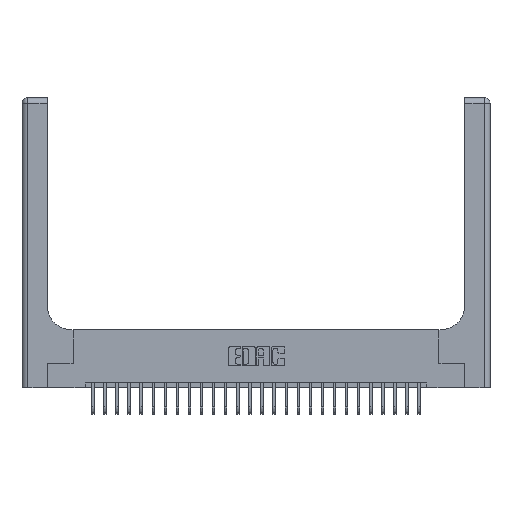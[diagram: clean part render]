
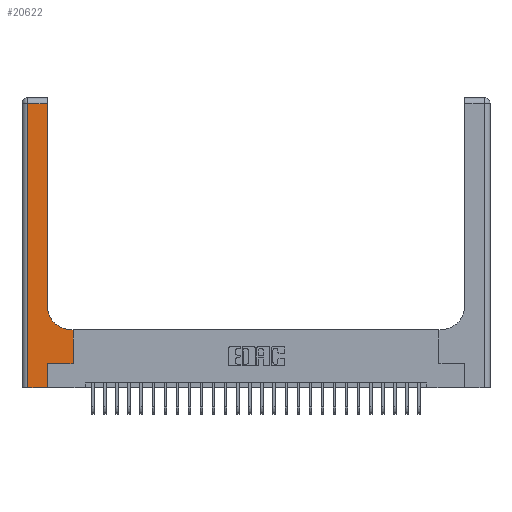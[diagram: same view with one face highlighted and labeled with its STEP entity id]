
A CAD part, top view. The second image highlights one B-rep face of the part: STEP entity #20622.
In plain terms, the highlighted planar face has unit normal (0, 0, 1).
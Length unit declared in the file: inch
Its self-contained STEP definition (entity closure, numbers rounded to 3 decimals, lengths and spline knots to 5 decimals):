
#846 = DIRECTION ( 'NONE',  ( 0., 1., 0. ) ) ;
#1114 = ORIENTED_EDGE ( 'NONE', *, *, #23028, .T. ) ;
#1119 = CARTESIAN_POINT ( 'NONE',  ( 0.528, 0.25, 0.37 ) ) ;
#1219 = VERTEX_POINT ( 'NONE', #4913 ) ;
#1459 = DIRECTION ( 'NONE',  ( -1., 0., 0. ) ) ;
#1529 = VECTOR ( 'NONE', #24369, 39.37008 ) ;
#1841 = CARTESIAN_POINT ( 'NONE',  ( 0.06, 3., 0.37 ) ) ;
#2082 = CARTESIAN_POINT ( 'NONE',  ( 0.528, 0.25, 0.37 ) ) ;
#2183 = AXIS2_PLACEMENT_3D ( 'NONE', #10645, #23799, #12576 ) ;
#2284 = LINE ( 'NONE', #24135, #16318 ) ;
#2545 = VERTEX_POINT ( 'NONE', #14846 ) ;
#2704 = AXIS2_PLACEMENT_3D ( 'NONE', #14211, #2793, #16126 ) ;
#2793 = DIRECTION ( 'NONE',  ( 0., 0., -1. ) ) ;
#3782 = DIRECTION ( 'NONE',  ( 0., -1., 0. ) ) ;
#3996 = EDGE_CURVE ( 'NONE', #2545, #10457, #22700, .T. ) ;
#4897 = CARTESIAN_POINT ( 'NONE',  ( 0.26, 0.85, 0.37 ) ) ;
#4913 = CARTESIAN_POINT ( 'NONE',  ( 0.06, 2.94, 0.37 ) ) ;
#5223 = ORIENTED_EDGE ( 'NONE', *, *, #15168, .T. ) ;
#5311 = LINE ( 'NONE', #9800, #19837 ) ;
#6964 = VECTOR ( 'NONE', #3782, 39.37008 ) ;
#7145 = FACE_OUTER_BOUND ( 'NONE', #19048, .T. ) ;
#7819 = CARTESIAN_POINT ( 'NONE',  ( 0.265, 0., 0.37 ) ) ;
#8802 = DIRECTION ( 'NONE',  ( 0., 1., 0. ) ) ;
#8806 = ORIENTED_EDGE ( 'NONE', *, *, #12854, .T. ) ;
#9182 = VECTOR ( 'NONE', #846, 39.37008 ) ;
#9800 = CARTESIAN_POINT ( 'NONE',  ( 0., 0., 0.37 ) ) ;
#10286 = VERTEX_POINT ( 'NONE', #23382 ) ;
#10457 = VERTEX_POINT ( 'NONE', #10545 ) ;
#10545 = CARTESIAN_POINT ( 'NONE',  ( 0.265, 0.25, 0.37 ) ) ;
#10645 = CARTESIAN_POINT ( 'NONE',  ( 0., 3., 0.37 ) ) ;
#11180 = CARTESIAN_POINT ( 'NONE',  ( 0.528, 0.6, 0.37 ) ) ;
#11387 = VERTEX_POINT ( 'NONE', #2082 ) ;
#11705 = VERTEX_POINT ( 'NONE', #18222 ) ;
#11707 = LINE ( 'NONE', #22487, #1529 ) ;
#12102 = LINE ( 'NONE', #16204, #16572 ) ;
#12576 = DIRECTION ( 'NONE',  ( -1., 0., 0. ) ) ;
#12854 = EDGE_CURVE ( 'NONE', #1219, #21657, #22038, .T. ) ;
#14211 = CARTESIAN_POINT ( 'NONE',  ( 0.51, 0.85, 0.37 ) ) ;
#14584 = EDGE_CURVE ( 'NONE', #11387, #23557, #16471, .T. ) ;
#14768 = EDGE_CURVE ( 'NONE', #10457, #11387, #11707, .T. ) ;
#14846 = CARTESIAN_POINT ( 'NONE',  ( 0.265, 0., 0.37 ) ) ;
#15168 = EDGE_CURVE ( 'NONE', #23996, #11705, #24209, .T. ) ;
#15738 = ORIENTED_EDGE ( 'NONE', *, *, #24145, .T. ) ;
#15866 = VECTOR ( 'NONE', #8802, 39.37008 ) ;
#16104 = CARTESIAN_POINT ( 'NONE',  ( 0.06, 0., 0.37 ) ) ;
#16126 = DIRECTION ( 'NONE',  ( 1., 0., 0. ) ) ;
#16204 = CARTESIAN_POINT ( 'NONE',  ( 0., 2.94, 0.37 ) ) ;
#16318 = VECTOR ( 'NONE', #1459, 39.37008 ) ;
#16471 = LINE ( 'NONE', #1119, #15866 ) ;
#16572 = VECTOR ( 'NONE', #18092, 39.37008 ) ;
#17132 = EDGE_CURVE ( 'NONE', #11705, #1219, #12102, .T. ) ;
#17168 = VECTOR ( 'NONE', #22909, 39.37008 ) ;
#17465 = DIRECTION ( 'NONE',  ( 1., 0., 0. ) ) ;
#18092 = DIRECTION ( 'NONE',  ( -1., 0., 0. ) ) ;
#18222 = CARTESIAN_POINT ( 'NONE',  ( 0.26, 2.94, 0.37 ) ) ;
#18322 = ORIENTED_EDGE ( 'NONE', *, *, #17132, .T. ) ;
#18592 = ORIENTED_EDGE ( 'NONE', *, *, #14584, .T. ) ;
#19048 = EDGE_LOOP ( 'NONE', ( #5223, #18322, #8806, #20365, #20625, #22366, #18592, #15738, #1114 ) ) ;
#19837 = VECTOR ( 'NONE', #17465, 39.37008 ) ;
#20116 = CIRCLE ( 'NONE', #2704, 0.25 ) ;
#20365 = ORIENTED_EDGE ( 'NONE', *, *, #22852, .T. ) ;
#20622 = ADVANCED_FACE ( 'NONE', ( #7145 ), #21936, .F. ) ;
#20625 = ORIENTED_EDGE ( 'NONE', *, *, #3996, .T. ) ;
#21657 = VERTEX_POINT ( 'NONE', #16104 ) ;
#21936 = PLANE ( 'NONE',  #2183 ) ;
#22038 = LINE ( 'NONE', #1841, #6964 ) ;
#22366 = ORIENTED_EDGE ( 'NONE', *, *, #14768, .T. ) ;
#22487 = CARTESIAN_POINT ( 'NONE',  ( 0.265, 0.25, 0.37 ) ) ;
#22700 = LINE ( 'NONE', #7819, #17168 ) ;
#22852 = EDGE_CURVE ( 'NONE', #21657, #2545, #5311, .T. ) ;
#22909 = DIRECTION ( 'NONE',  ( 0., 1., 0. ) ) ;
#23028 = EDGE_CURVE ( 'NONE', #10286, #23996, #20116, .T. ) ;
#23382 = CARTESIAN_POINT ( 'NONE',  ( 0.51, 0.6, 0.37 ) ) ;
#23515 = CARTESIAN_POINT ( 'NONE',  ( 0.26, 3., 0.37 ) ) ;
#23557 = VERTEX_POINT ( 'NONE', #11180 ) ;
#23799 = DIRECTION ( 'NONE',  ( 0., 0., -1. ) ) ;
#23996 = VERTEX_POINT ( 'NONE', #4897 ) ;
#24135 = CARTESIAN_POINT ( 'NONE',  ( 0.26, 0.6, 0.37 ) ) ;
#24145 = EDGE_CURVE ( 'NONE', #23557, #10286, #2284, .T. ) ;
#24209 = LINE ( 'NONE', #23515, #9182 ) ;
#24369 = DIRECTION ( 'NONE',  ( 1., 0., 0. ) ) ;
